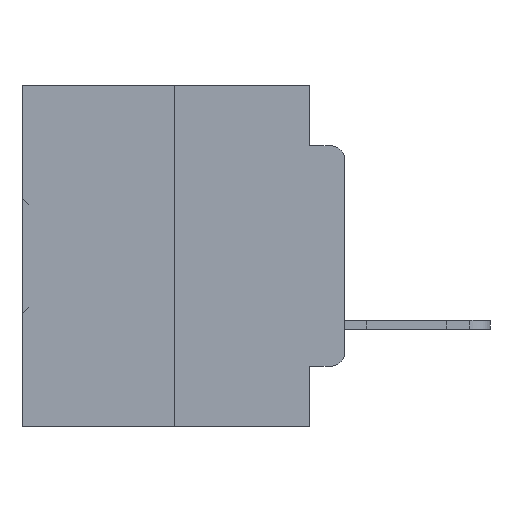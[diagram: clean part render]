
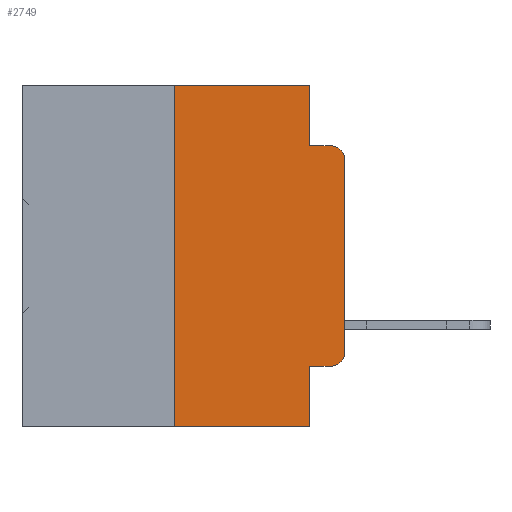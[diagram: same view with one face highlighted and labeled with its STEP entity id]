
A CAD part, left-side view. The second image highlights one B-rep face of the part: STEP entity #2749.
In plain terms, the highlighted planar face has unit normal (-1, 0, 0).
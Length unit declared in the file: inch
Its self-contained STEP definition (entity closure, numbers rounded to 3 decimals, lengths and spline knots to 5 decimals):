
#212 = CIRCLE ( 'NONE', #2968, 0.02 ) ;
#567 = ORIENTED_EDGE ( 'NONE', *, *, #1168, .T. ) ;
#814 = ORIENTED_EDGE ( 'NONE', *, *, #24202, .T. ) ;
#822 = ORIENTED_EDGE ( 'NONE', *, *, #10460, .T. ) ;
#1168 = EDGE_CURVE ( 'NONE', #16337, #26299, #18677, .T. ) ;
#1647 = VERTEX_POINT ( 'NONE', #11606 ) ;
#1751 = EDGE_LOOP ( 'NONE', ( #822, #2172, #5215, #5270, #28224, #28666, #567, #5563, #814, #8189 ) ) ;
#1893 = VECTOR ( 'NONE', #13614, 39.37008 ) ;
#1979 = VERTEX_POINT ( 'NONE', #7192 ) ;
#2172 = ORIENTED_EDGE ( 'NONE', *, *, #10735, .T. ) ;
#2749 = ADVANCED_FACE ( 'NONE', ( #31346 ), #19565, .F. ) ;
#2968 = AXIS2_PLACEMENT_3D ( 'NONE', #31777, #31746, #31737 ) ;
#4245 = VECTOR ( 'NONE', #7898, 39.37008 ) ;
#5215 = ORIENTED_EDGE ( 'NONE', *, *, #10781, .F. ) ;
#5270 = ORIENTED_EDGE ( 'NONE', *, *, #11394, .F. ) ;
#5563 = ORIENTED_EDGE ( 'NONE', *, *, #23909, .F. ) ;
#6374 = DIRECTION ( 'NONE',  ( 1., 0., 0. ) ) ;
#6445 = DIRECTION ( 'NONE',  ( 0., 0., -1. ) ) ;
#6588 = CARTESIAN_POINT ( 'NONE',  ( 0., 0.02, -0.0885 ) ) ;
#7192 = CARTESIAN_POINT ( 'NONE',  ( 0., 0.25, 0. ) ) ;
#7317 = LINE ( 'NONE', #31815, #14866 ) ;
#7736 = CARTESIAN_POINT ( 'NONE',  ( 0., 0.25, -0.5 ) ) ;
#7841 = VECTOR ( 'NONE', #11424, 39.37008 ) ;
#7898 = DIRECTION ( 'NONE',  ( 0., -1., 0. ) ) ;
#8189 = ORIENTED_EDGE ( 'NONE', *, *, #24290, .T. ) ;
#8410 = CARTESIAN_POINT ( 'NONE',  ( 0., 0.02, -0.3915 ) ) ;
#9776 = LINE ( 'NONE', #14103, #1893 ) ;
#10460 = EDGE_CURVE ( 'NONE', #27325, #11621, #35123, .T. ) ;
#10664 = AXIS2_PLACEMENT_3D ( 'NONE', #17048, #6374, #6445 ) ;
#10735 = EDGE_CURVE ( 'NONE', #11621, #17987, #212, .T. ) ;
#10781 = EDGE_CURVE ( 'NONE', #22298, #17987, #7317, .T. ) ;
#11280 = DIRECTION ( 'NONE',  ( 0., 0., -1. ) ) ;
#11394 = EDGE_CURVE ( 'NONE', #31280, #22298, #13083, .T. ) ;
#11424 = DIRECTION ( 'NONE',  ( 0., -1., 0. ) ) ;
#11606 = CARTESIAN_POINT ( 'NONE',  ( 0., 0.051, -0.4115 ) ) ;
#11621 = VERTEX_POINT ( 'NONE', #20925 ) ;
#13083 = LINE ( 'NONE', #24043, #25454 ) ;
#13582 = VECTOR ( 'NONE', #34145, 39.37008 ) ;
#13614 = DIRECTION ( 'NONE',  ( 0., 0., 1. ) ) ;
#14103 = CARTESIAN_POINT ( 'NONE',  ( 0., 0.25, 0. ) ) ;
#14866 = VECTOR ( 'NONE', #31516, 39.37008 ) ;
#15355 = LINE ( 'NONE', #30677, #7841 ) ;
#15439 = EDGE_CURVE ( 'NONE', #16337, #1979, #9776, .T. ) ;
#16337 = VERTEX_POINT ( 'NONE', #7736 ) ;
#16848 = VECTOR ( 'NONE', #26614, 39.37008 ) ;
#17048 = CARTESIAN_POINT ( 'NONE',  ( 0., 0.473, 0. ) ) ;
#17539 = AXIS2_PLACEMENT_3D ( 'NONE', #8410, #27956, #11280 ) ;
#17987 = VERTEX_POINT ( 'NONE', #6588 ) ;
#18677 = LINE ( 'NONE', #31078, #16848 ) ;
#19565 = PLANE ( 'NONE',  #10664 ) ;
#20006 = CARTESIAN_POINT ( 'NONE',  ( 0., 0.051, 0. ) ) ;
#20925 = CARTESIAN_POINT ( 'NONE',  ( 0., 0., -0.1085 ) ) ;
#20958 = CARTESIAN_POINT ( 'NONE',  ( 0., 0.051, 0. ) ) ;
#20985 = VECTOR ( 'NONE', #34132, 39.37008 ) ;
#21940 = CARTESIAN_POINT ( 'NONE',  ( 0., 0., -0.3915 ) ) ;
#22298 = VERTEX_POINT ( 'NONE', #33005 ) ;
#22621 = CARTESIAN_POINT ( 'NONE',  ( 0., 0.02, -0.4115 ) ) ;
#23474 = CARTESIAN_POINT ( 'NONE',  ( 0., 0.051, -0.5 ) ) ;
#23742 = DIRECTION ( 'NONE',  ( 0., 0., -1. ) ) ;
#23909 = EDGE_CURVE ( 'NONE', #1647, #26299, #28111, .T. ) ;
#24043 = CARTESIAN_POINT ( 'NONE',  ( 0., 0.051, 0. ) ) ;
#24202 = EDGE_CURVE ( 'NONE', #1647, #32655, #33709, .T. ) ;
#24290 = EDGE_CURVE ( 'NONE', #32655, #27325, #24426, .T. ) ;
#24426 = CIRCLE ( 'NONE', #17539, 0.02 ) ;
#25454 = VECTOR ( 'NONE', #23742, 39.37008 ) ;
#26299 = VERTEX_POINT ( 'NONE', #23474 ) ;
#26614 = DIRECTION ( 'NONE',  ( 0., -1., 0. ) ) ;
#27325 = VERTEX_POINT ( 'NONE', #21940 ) ;
#27956 = DIRECTION ( 'NONE',  ( -1., 0., 0. ) ) ;
#28111 = LINE ( 'NONE', #20958, #20985 ) ;
#28224 = ORIENTED_EDGE ( 'NONE', *, *, #30037, .F. ) ;
#28666 = ORIENTED_EDGE ( 'NONE', *, *, #15439, .F. ) ;
#30037 = EDGE_CURVE ( 'NONE', #1979, #31280, #15355, .T. ) ;
#30677 = CARTESIAN_POINT ( 'NONE',  ( 0., 0.473, 0. ) ) ;
#31078 = CARTESIAN_POINT ( 'NONE',  ( 0., 0.473, -0.5 ) ) ;
#31280 = VERTEX_POINT ( 'NONE', #20006 ) ;
#31346 = FACE_OUTER_BOUND ( 'NONE', #1751, .T. ) ;
#31516 = DIRECTION ( 'NONE',  ( 0., -1., 0. ) ) ;
#31737 = DIRECTION ( 'NONE',  ( 0., 0., -1. ) ) ;
#31746 = DIRECTION ( 'NONE',  ( -1., 0., 0. ) ) ;
#31777 = CARTESIAN_POINT ( 'NONE',  ( 0., 0.02, -0.1085 ) ) ;
#31815 = CARTESIAN_POINT ( 'NONE',  ( 0., 0.051, -0.0885 ) ) ;
#32655 = VERTEX_POINT ( 'NONE', #22621 ) ;
#33005 = CARTESIAN_POINT ( 'NONE',  ( 0., 0.051, -0.0885 ) ) ;
#33709 = LINE ( 'NONE', #35091, #4245 ) ;
#34132 = DIRECTION ( 'NONE',  ( 0., 0., -1. ) ) ;
#34145 = DIRECTION ( 'NONE',  ( 0., 0., 1. ) ) ;
#34550 = CARTESIAN_POINT ( 'NONE',  ( 0., 0., 0. ) ) ;
#35091 = CARTESIAN_POINT ( 'NONE',  ( 0., 0.051, -0.4115 ) ) ;
#35123 = LINE ( 'NONE', #34550, #13582 ) ;
